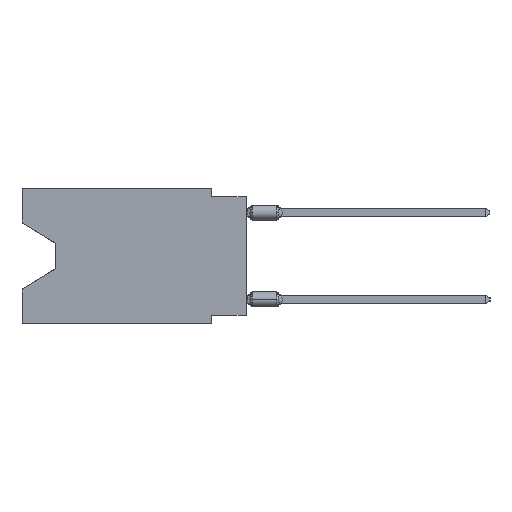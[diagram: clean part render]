
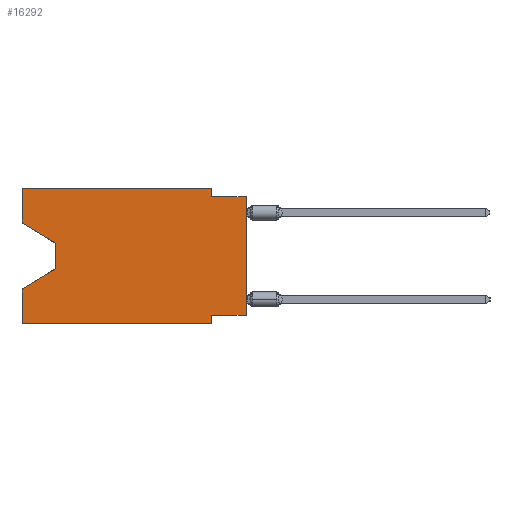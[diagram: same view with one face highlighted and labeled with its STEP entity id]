
A CAD part, left-side view. The second image highlights one B-rep face of the part: STEP entity #16292.
In plain terms, the highlighted planar face has unit normal (-1, 0, 0).
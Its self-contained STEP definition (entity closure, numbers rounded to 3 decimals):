
#1640 = EDGE_CURVE ( 'NONE', #7677, #33657, #31761, .T. ) ;
#2877 = LINE ( 'NONE', #32722, #32372 ) ;
#3286 = VECTOR ( 'NONE', #49463, 1000. ) ;
#3741 = ORIENTED_EDGE ( 'NONE', *, *, #55222, .F. ) ;
#4520 = VERTEX_POINT ( 'NONE', #25883 ) ;
#4760 = DIRECTION ( 'NONE',  ( 0., 0., -1. ) ) ;
#6711 = LINE ( 'NONE', #46727, #3286 ) ;
#6824 = DIRECTION ( 'NONE',  ( 0., -1., 0. ) ) ;
#7104 = ORIENTED_EDGE ( 'NONE', *, *, #60190, .F. ) ;
#7677 = VERTEX_POINT ( 'NONE', #53996 ) ;
#7941 = DIRECTION ( 'NONE',  ( 1., 0., 0. ) ) ;
#8065 = DIRECTION ( 'NONE',  ( 0., 0., -1. ) ) ;
#9358 = LINE ( 'NONE', #29384, #21262 ) ;
#10068 = CARTESIAN_POINT ( 'NONE',  ( 0., 16.383, 0. ) ) ;
#10226 = VECTOR ( 'NONE', #44672, 1000. ) ;
#13024 = DIRECTION ( 'NONE',  ( 0., 0., 1. ) ) ;
#13125 = CARTESIAN_POINT ( 'NONE',  ( 0., 0., -9.271 ) ) ;
#14046 = EDGE_CURVE ( 'NONE', #62148, #30110, #49905, .T. ) ;
#14865 = LINE ( 'NONE', #40446, #54509 ) ;
#16292 = ADVANCED_FACE ( 'NONE', ( #61426 ), #37478, .F. ) ;
#17021 = ORIENTED_EDGE ( 'NONE', *, *, #61786, .T. ) ;
#18060 = CARTESIAN_POINT ( 'NONE',  ( 0., 13.97, -4.013 ) ) ;
#19098 = CARTESIAN_POINT ( 'NONE',  ( 0., 0., -9.271 ) ) ;
#19182 = VECTOR ( 'NONE', #28890, 1000. ) ;
#19534 = CARTESIAN_POINT ( 'NONE',  ( 0., 2.54, -9.906 ) ) ;
#21262 = VECTOR ( 'NONE', #4760, 1000. ) ;
#22170 = EDGE_LOOP ( 'NONE', ( #40408, #17021, #57946, #56721, #48076, #55975, #7104, #46675, #29458, #46836, #47455, #3741 ) ) ;
#24381 = CARTESIAN_POINT ( 'NONE',  ( 0., 13.97, -5.893 ) ) ;
#24513 = DIRECTION ( 'NONE',  ( 0., 0., 1. ) ) ;
#25536 = CARTESIAN_POINT ( 'NONE',  ( 0., 2.54, 0. ) ) ;
#25883 = CARTESIAN_POINT ( 'NONE',  ( 0., 16.383, -7.36 ) ) ;
#26200 = CARTESIAN_POINT ( 'NONE',  ( 0., 16.383, -9.906 ) ) ;
#26979 = CARTESIAN_POINT ( 'NONE',  ( 0., 16.383, 0. ) ) ;
#27777 = CARTESIAN_POINT ( 'NONE',  ( 0., 13.97, -4.013 ) ) ;
#28890 = DIRECTION ( 'NONE',  ( 0., 0., -1. ) ) ;
#29384 = CARTESIAN_POINT ( 'NONE',  ( 0., 2.54, 0. ) ) ;
#29458 = ORIENTED_EDGE ( 'NONE', *, *, #45105, .F. ) ;
#30094 = LINE ( 'NONE', #39610, #58341 ) ;
#30110 = VERTEX_POINT ( 'NONE', #25536 ) ;
#30527 = VERTEX_POINT ( 'NONE', #62096 ) ;
#31761 = LINE ( 'NONE', #26200, #39400 ) ;
#32372 = VECTOR ( 'NONE', #13024, 1000. ) ;
#32722 = CARTESIAN_POINT ( 'NONE',  ( 0., 0., 0. ) ) ;
#33657 = VERTEX_POINT ( 'NONE', #19534 ) ;
#34872 = DIRECTION ( 'NONE',  ( 0., 0.855, -0.519 ) ) ;
#36738 = CARTESIAN_POINT ( 'NONE',  ( 0., 2.54, -9.271 ) ) ;
#37478 = PLANE ( 'NONE',  #38513 ) ;
#38478 = LINE ( 'NONE', #19098, #56823 ) ;
#38513 = AXIS2_PLACEMENT_3D ( 'NONE', #26979, #7941, #46994 ) ;
#39400 = VECTOR ( 'NONE', #6824, 1000. ) ;
#39610 = CARTESIAN_POINT ( 'NONE',  ( 0., 16.383, 0. ) ) ;
#40408 = ORIENTED_EDGE ( 'NONE', *, *, #63175, .T. ) ;
#40446 = CARTESIAN_POINT ( 'NONE',  ( 0., 13.97, -5.893 ) ) ;
#41225 = VECTOR ( 'NONE', #24513, 1000. ) ;
#41895 = EDGE_CURVE ( 'NONE', #49520, #48395, #2877, .T. ) ;
#42684 = CARTESIAN_POINT ( 'NONE',  ( 0., 2.54, -9.906 ) ) ;
#43565 = EDGE_CURVE ( 'NONE', #45349, #4520, #14865, .T. ) ;
#44672 = DIRECTION ( 'NONE',  ( 0., -1., 0. ) ) ;
#45105 = EDGE_CURVE ( 'NONE', #30527, #48395, #6711, .T. ) ;
#45349 = VERTEX_POINT ( 'NONE', #24381 ) ;
#45427 = LINE ( 'NONE', #64147, #60033 ) ;
#46675 = ORIENTED_EDGE ( 'NONE', *, *, #41895, .T. ) ;
#46727 = CARTESIAN_POINT ( 'NONE',  ( 0., 0., -0.635 ) ) ;
#46836 = ORIENTED_EDGE ( 'NONE', *, *, #60874, .F. ) ;
#46994 = DIRECTION ( 'NONE',  ( 0., 0., -1. ) ) ;
#47048 = VERTEX_POINT ( 'NONE', #59396 ) ;
#47455 = ORIENTED_EDGE ( 'NONE', *, *, #14046, .F. ) ;
#48076 = ORIENTED_EDGE ( 'NONE', *, *, #1640, .T. ) ;
#48395 = VERTEX_POINT ( 'NONE', #58806 ) ;
#48730 = VERTEX_POINT ( 'NONE', #18060 ) ;
#48749 = EDGE_CURVE ( 'NONE', #50713, #33657, #53170, .T. ) ;
#49066 = DIRECTION ( 'NONE',  ( 0., -0.855, -0.519 ) ) ;
#49125 = LINE ( 'NONE', #10068, #41225 ) ;
#49463 = DIRECTION ( 'NONE',  ( 0., -1., 0. ) ) ;
#49520 = VERTEX_POINT ( 'NONE', #13125 ) ;
#49905 = LINE ( 'NONE', #55810, #10226 ) ;
#50098 = DIRECTION ( 'NONE',  ( 0., 0., 1. ) ) ;
#50713 = VERTEX_POINT ( 'NONE', #36738 ) ;
#53170 = LINE ( 'NONE', #42684, #19182 ) ;
#53996 = CARTESIAN_POINT ( 'NONE',  ( 0., 16.383, -9.906 ) ) ;
#54509 = VECTOR ( 'NONE', #34872, 1000. ) ;
#54544 = DIRECTION ( 'NONE',  ( 0., 1., 0. ) ) ;
#55222 = EDGE_CURVE ( 'NONE', #47048, #62148, #30094, .T. ) ;
#55810 = CARTESIAN_POINT ( 'NONE',  ( 0., 16.383, 0. ) ) ;
#55975 = ORIENTED_EDGE ( 'NONE', *, *, #48749, .F. ) ;
#56721 = ORIENTED_EDGE ( 'NONE', *, *, #61501, .F. ) ;
#56823 = VECTOR ( 'NONE', #54544, 1000. ) ;
#57946 = ORIENTED_EDGE ( 'NONE', *, *, #43565, .T. ) ;
#58341 = VECTOR ( 'NONE', #50098, 1000. ) ;
#58583 = LINE ( 'NONE', #27777, #64294 ) ;
#58806 = CARTESIAN_POINT ( 'NONE',  ( 0., 0., -0.635 ) ) ;
#59396 = CARTESIAN_POINT ( 'NONE',  ( 0., 16.383, -2.546 ) ) ;
#60033 = VECTOR ( 'NONE', #49066, 1000. ) ;
#60190 = EDGE_CURVE ( 'NONE', #49520, #50713, #38478, .T. ) ;
#60874 = EDGE_CURVE ( 'NONE', #30110, #30527, #9358, .T. ) ;
#61426 = FACE_OUTER_BOUND ( 'NONE', #22170, .T. ) ;
#61501 = EDGE_CURVE ( 'NONE', #7677, #4520, #49125, .T. ) ;
#61786 = EDGE_CURVE ( 'NONE', #48730, #45349, #58583, .T. ) ;
#62096 = CARTESIAN_POINT ( 'NONE',  ( 0., 2.54, -0.635 ) ) ;
#62138 = CARTESIAN_POINT ( 'NONE',  ( 0., 16.383, 0. ) ) ;
#62148 = VERTEX_POINT ( 'NONE', #62138 ) ;
#63175 = EDGE_CURVE ( 'NONE', #47048, #48730, #45427, .T. ) ;
#64147 = CARTESIAN_POINT ( 'NONE',  ( 0., 16.383, -2.546 ) ) ;
#64294 = VECTOR ( 'NONE', #8065, 1000. ) ;
